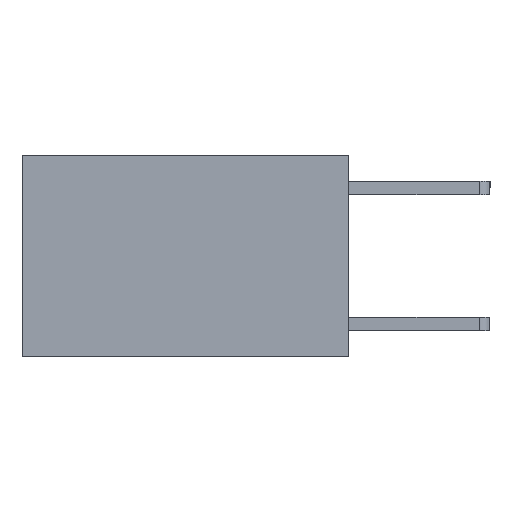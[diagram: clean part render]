
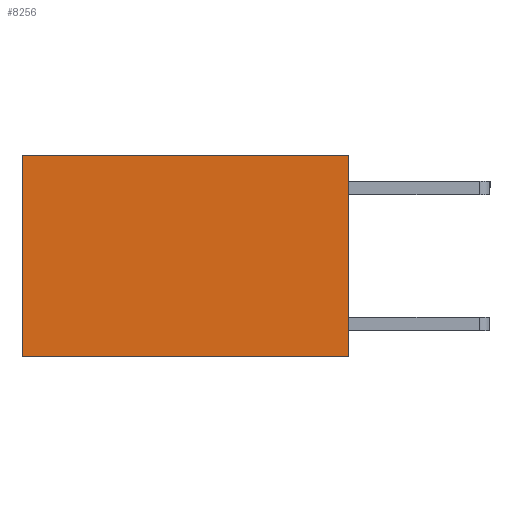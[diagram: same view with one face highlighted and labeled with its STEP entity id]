
A CAD part, left-side view. The second image highlights one B-rep face of the part: STEP entity #8256.
In plain terms, the highlighted planar face has unit normal (-1, 0, 0).
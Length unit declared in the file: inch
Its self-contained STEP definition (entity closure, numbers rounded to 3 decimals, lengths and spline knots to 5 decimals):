
#228 = LINE ( 'NONE', #3806, #2544 ) ;
#627 = VECTOR ( 'NONE', #1719, 39.37008 ) ;
#761 = LINE ( 'NONE', #4167, #6242 ) ;
#1413 = CARTESIAN_POINT ( 'NONE',  ( 0.2625, 0., 0. ) ) ;
#1719 = DIRECTION ( 'NONE',  ( 0., 1., 0. ) ) ;
#2060 = ORIENTED_EDGE ( 'NONE', *, *, #2843, .F. ) ;
#2425 = EDGE_CURVE ( 'NONE', #7168, #10334, #2603, .T. ) ;
#2544 = VECTOR ( 'NONE', #9334, 39.37008 ) ;
#2603 = LINE ( 'NONE', #9732, #627 ) ;
#2843 = EDGE_CURVE ( 'NONE', #10756, #10650, #761, .T. ) ;
#2856 = EDGE_CURVE ( 'NONE', #7168, #10756, #10413, .T. ) ;
#3234 = DIRECTION ( 'NONE',  ( 0., 1., 0. ) ) ;
#3806 = CARTESIAN_POINT ( 'NONE',  ( 0.2625, 0.6, 0. ) ) ;
#4167 = CARTESIAN_POINT ( 'NONE',  ( 0.2625, 0., -0.37 ) ) ;
#5136 = EDGE_CURVE ( 'NONE', #10334, #10650, #228, .T. ) ;
#5154 = CARTESIAN_POINT ( 'NONE',  ( 0.2625, 0., 0. ) ) ;
#5340 = ORIENTED_EDGE ( 'NONE', *, *, #5136, .T. ) ;
#5645 = EDGE_LOOP ( 'NONE', ( #5340, #2060, #8261, #10311 ) ) ;
#6139 = PLANE ( 'NONE',  #8400 ) ;
#6242 = VECTOR ( 'NONE', #3234, 39.37008 ) ;
#7168 = VERTEX_POINT ( 'NONE', #10808 ) ;
#8256 = ADVANCED_FACE ( 'NONE', ( #9591 ), #6139, .F. ) ;
#8261 = ORIENTED_EDGE ( 'NONE', *, *, #2856, .F. ) ;
#8400 = AXIS2_PLACEMENT_3D ( 'NONE', #5154, #9473, #11334 ) ;
#8658 = VECTOR ( 'NONE', #11450, 39.37008 ) ;
#9334 = DIRECTION ( 'NONE',  ( 0., 0., -1. ) ) ;
#9473 = DIRECTION ( 'NONE',  ( 1., 0., 0. ) ) ;
#9591 = FACE_OUTER_BOUND ( 'NONE', #5645, .T. ) ;
#9732 = CARTESIAN_POINT ( 'NONE',  ( 0.2625, 0., 0. ) ) ;
#10311 = ORIENTED_EDGE ( 'NONE', *, *, #2425, .T. ) ;
#10334 = VERTEX_POINT ( 'NONE', #10734 ) ;
#10413 = LINE ( 'NONE', #1413, #8658 ) ;
#10650 = VERTEX_POINT ( 'NONE', #10791 ) ;
#10734 = CARTESIAN_POINT ( 'NONE',  ( 0.2625, 0.6, 0. ) ) ;
#10756 = VERTEX_POINT ( 'NONE', #11188 ) ;
#10791 = CARTESIAN_POINT ( 'NONE',  ( 0.2625, 0.6, -0.37 ) ) ;
#10808 = CARTESIAN_POINT ( 'NONE',  ( 0.2625, 0., 0. ) ) ;
#11188 = CARTESIAN_POINT ( 'NONE',  ( 0.2625, 0., -0.37 ) ) ;
#11334 = DIRECTION ( 'NONE',  ( 0., 0., -1. ) ) ;
#11450 = DIRECTION ( 'NONE',  ( 0., 0., -1. ) ) ;
